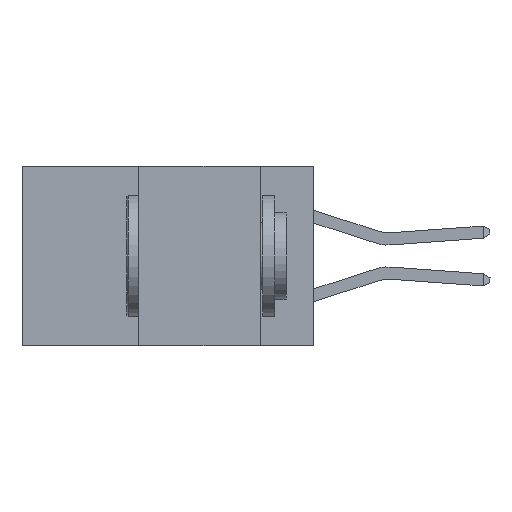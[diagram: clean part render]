
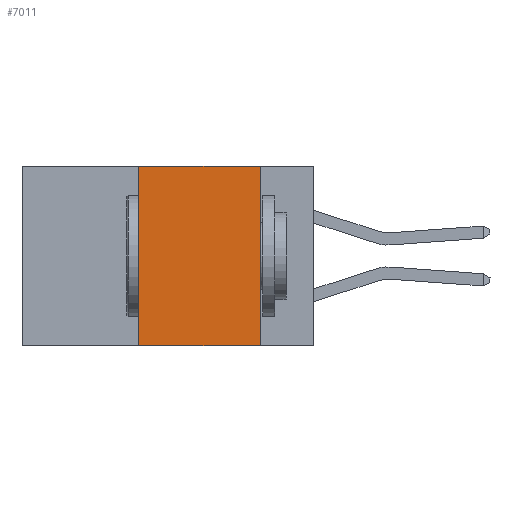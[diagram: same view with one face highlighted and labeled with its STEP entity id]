
A CAD part, left-side view. The second image highlights one B-rep face of the part: STEP entity #7011.
In plain terms, the highlighted planar face has unit normal (-1, 0, 0).
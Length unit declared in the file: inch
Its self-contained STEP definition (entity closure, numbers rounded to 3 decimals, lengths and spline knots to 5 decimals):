
#213 = ORIENTED_EDGE ( 'NONE', *, *, #18521, .T. ) ;
#795 = EDGE_CURVE ( 'NONE', #16112, #9826, #16115, .T. ) ;
#2889 = EDGE_LOOP ( 'NONE', ( #20525, #4364, #9560, #213 ) ) ;
#3595 = EDGE_CURVE ( 'NONE', #15930, #9172, #21802, .T. ) ;
#4364 = ORIENTED_EDGE ( 'NONE', *, *, #8625, .F. ) ;
#4420 = CARTESIAN_POINT ( 'NONE',  ( 0., 0.36, -0.37 ) ) ;
#5025 = VECTOR ( 'NONE', #16554, 39.37008 ) ;
#5276 = CARTESIAN_POINT ( 'NONE',  ( 0., 0.36, 0. ) ) ;
#5609 = CARTESIAN_POINT ( 'NONE',  ( 0., 0.6, -0.37 ) ) ;
#6449 = CARTESIAN_POINT ( 'NONE',  ( 0., 0.11, 0. ) ) ;
#6507 = AXIS2_PLACEMENT_3D ( 'NONE', #19209, #11533, #9444 ) ;
#7011 = ADVANCED_FACE ( 'NONE', ( #24712 ), #23056, .F. ) ;
#8625 = EDGE_CURVE ( 'NONE', #9172, #16112, #10677, .T. ) ;
#9172 = VERTEX_POINT ( 'NONE', #5276 ) ;
#9444 = DIRECTION ( 'NONE',  ( 0., 0., -1. ) ) ;
#9560 = ORIENTED_EDGE ( 'NONE', *, *, #3595, .F. ) ;
#9826 = VERTEX_POINT ( 'NONE', #23754 ) ;
#10677 = LINE ( 'NONE', #13166, #18666 ) ;
#11533 = DIRECTION ( 'NONE',  ( 1., 0., 0. ) ) ;
#11965 = DIRECTION ( 'NONE',  ( 0., -1., 0. ) ) ;
#13166 = CARTESIAN_POINT ( 'NONE',  ( 0., 0.6, 0. ) ) ;
#15930 = VERTEX_POINT ( 'NONE', #4420 ) ;
#16112 = VERTEX_POINT ( 'NONE', #22994 ) ;
#16115 = LINE ( 'NONE', #6449, #20740 ) ;
#16554 = DIRECTION ( 'NONE',  ( 0., -1., 0. ) ) ;
#18261 = DIRECTION ( 'NONE',  ( 0., 0., -1. ) ) ;
#18521 = EDGE_CURVE ( 'NONE', #15930, #9826, #24996, .T. ) ;
#18666 = VECTOR ( 'NONE', #11965, 39.37008 ) ;
#19209 = CARTESIAN_POINT ( 'NONE',  ( 0., 0.6, 0. ) ) ;
#19729 = CARTESIAN_POINT ( 'NONE',  ( 0., 0.36, 0. ) ) ;
#20525 = ORIENTED_EDGE ( 'NONE', *, *, #795, .F. ) ;
#20740 = VECTOR ( 'NONE', #18261, 39.37008 ) ;
#21751 = DIRECTION ( 'NONE',  ( 0., 0., 1. ) ) ;
#21802 = LINE ( 'NONE', #19729, #24908 ) ;
#22994 = CARTESIAN_POINT ( 'NONE',  ( 0., 0.11, 0. ) ) ;
#23056 = PLANE ( 'NONE',  #6507 ) ;
#23754 = CARTESIAN_POINT ( 'NONE',  ( 0., 0.11, -0.37 ) ) ;
#24712 = FACE_OUTER_BOUND ( 'NONE', #2889, .T. ) ;
#24908 = VECTOR ( 'NONE', #21751, 39.37008 ) ;
#24996 = LINE ( 'NONE', #5609, #5025 ) ;
